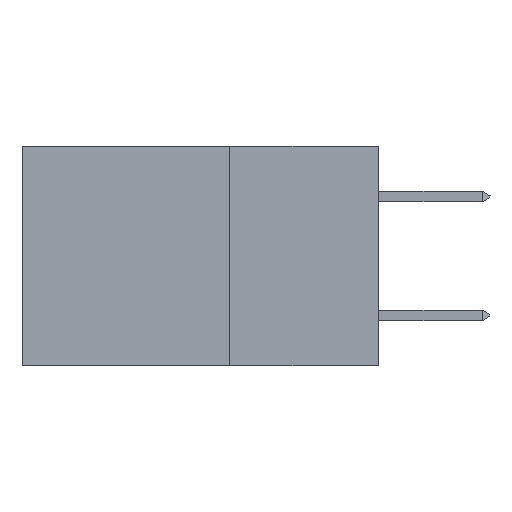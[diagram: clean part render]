
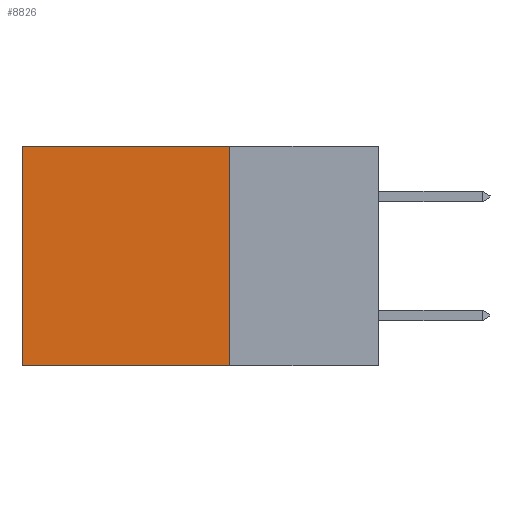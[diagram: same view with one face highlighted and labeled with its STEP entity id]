
A CAD part, left-side view. The second image highlights one B-rep face of the part: STEP entity #8826.
In plain terms, the highlighted planar face has unit normal (-1, 0, 0).
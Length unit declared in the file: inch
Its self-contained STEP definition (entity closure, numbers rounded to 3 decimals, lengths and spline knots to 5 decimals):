
#256 = ORIENTED_EDGE ( 'NONE', *, *, #8630, .T. ) ;
#691 = LINE ( 'NONE', #9605, #1444 ) ;
#1444 = VECTOR ( 'NONE', #5214, 39.37008 ) ;
#1840 = ORIENTED_EDGE ( 'NONE', *, *, #2324, .T. ) ;
#2324 = EDGE_CURVE ( 'NONE', #6617, #14775, #4347, .T. ) ;
#2490 = DIRECTION ( 'NONE',  ( 0., 0., -1. ) ) ;
#4194 = ORIENTED_EDGE ( 'NONE', *, *, #5626, .F. ) ;
#4234 = LINE ( 'NONE', #5445, #9842 ) ;
#4347 = LINE ( 'NONE', #7475, #12937 ) ;
#4357 = VERTEX_POINT ( 'NONE', #14961 ) ;
#4666 = CARTESIAN_POINT ( 'NONE',  ( 0.2615, 0.6, -0.37 ) ) ;
#4783 = DIRECTION ( 'NONE',  ( 0., 1., 0. ) ) ;
#5214 = DIRECTION ( 'NONE',  ( 0., 1., 0. ) ) ;
#5445 = CARTESIAN_POINT ( 'NONE',  ( 0.2615, 0.25, -0.37 ) ) ;
#5626 = EDGE_CURVE ( 'NONE', #7723, #14775, #691, .T. ) ;
#5823 = PLANE ( 'NONE',  #8057 ) ;
#5931 = LINE ( 'NONE', #12209, #10706 ) ;
#6485 = EDGE_LOOP ( 'NONE', ( #1840, #4194, #7234, #256 ) ) ;
#6617 = VERTEX_POINT ( 'NONE', #13125 ) ;
#7234 = ORIENTED_EDGE ( 'NONE', *, *, #11545, .F. ) ;
#7475 = CARTESIAN_POINT ( 'NONE',  ( 0.2615, 0.6, -0.37 ) ) ;
#7723 = VERTEX_POINT ( 'NONE', #12339 ) ;
#8022 = CARTESIAN_POINT ( 'NONE',  ( 0.2615, 0.25, -0.37 ) ) ;
#8057 = AXIS2_PLACEMENT_3D ( 'NONE', #8022, #12722, #2490 ) ;
#8321 = FACE_OUTER_BOUND ( 'NONE', #6485, .T. ) ;
#8630 = EDGE_CURVE ( 'NONE', #4357, #6617, #5931, .T. ) ;
#8826 = ADVANCED_FACE ( 'NONE', ( #8321 ), #5823, .F. ) ;
#9605 = CARTESIAN_POINT ( 'NONE',  ( 0.2615, 0.25, -0.37 ) ) ;
#9842 = VECTOR ( 'NONE', #9902, 39.37008 ) ;
#9902 = DIRECTION ( 'NONE',  ( 0., 0., -1. ) ) ;
#10706 = VECTOR ( 'NONE', #4783, 39.37008 ) ;
#11545 = EDGE_CURVE ( 'NONE', #4357, #7723, #4234, .T. ) ;
#12209 = CARTESIAN_POINT ( 'NONE',  ( 0.2615, 0.25, 0. ) ) ;
#12339 = CARTESIAN_POINT ( 'NONE',  ( 0.2615, 0.25, -0.37 ) ) ;
#12722 = DIRECTION ( 'NONE',  ( 1., 0., 0. ) ) ;
#12937 = VECTOR ( 'NONE', #14604, 39.37008 ) ;
#13125 = CARTESIAN_POINT ( 'NONE',  ( 0.2615, 0.6, 0. ) ) ;
#14604 = DIRECTION ( 'NONE',  ( 0., 0., -1. ) ) ;
#14775 = VERTEX_POINT ( 'NONE', #4666 ) ;
#14961 = CARTESIAN_POINT ( 'NONE',  ( 0.2615, 0.25, 0. ) ) ;
